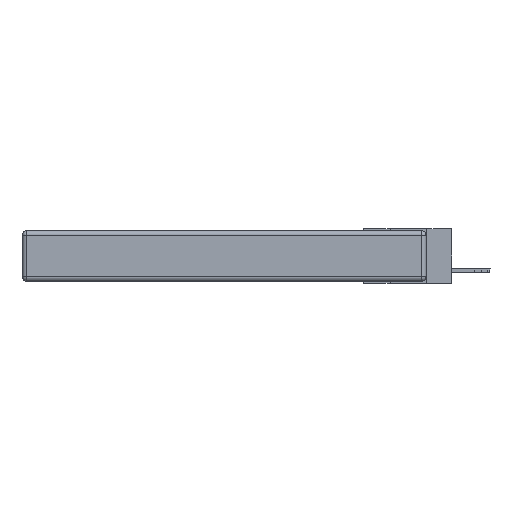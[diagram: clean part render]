
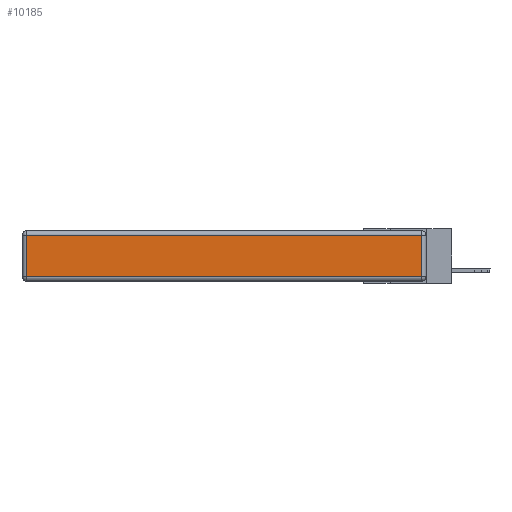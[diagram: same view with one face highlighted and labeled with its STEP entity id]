
A CAD part, left-side view. The second image highlights one B-rep face of the part: STEP entity #10185.
In plain terms, the highlighted planar face has unit normal (-1, 0, 0).
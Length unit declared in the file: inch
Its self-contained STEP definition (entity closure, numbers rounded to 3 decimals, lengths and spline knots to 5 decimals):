
#319 = LINE ( 'NONE', #3520, #14723 ) ;
#1107 = CARTESIAN_POINT ( 'NONE',  ( 0., 0., -0.343 ) ) ;
#1372 = ORIENTED_EDGE ( 'NONE', *, *, #13783, .T. ) ;
#1484 = VERTEX_POINT ( 'NONE', #5855 ) ;
#1899 = DIRECTION ( 'NONE',  ( 0., 0., 1. ) ) ;
#3520 = CARTESIAN_POINT ( 'NONE',  ( 0., 0., -0.313 ) ) ;
#4448 = FACE_OUTER_BOUND ( 'NONE', #14751, .T. ) ;
#4524 = VECTOR ( 'NONE', #13594, 39.37008 ) ;
#5392 = ORIENTED_EDGE ( 'NONE', *, *, #12137, .T. ) ;
#5855 = CARTESIAN_POINT ( 'NONE',  ( 0., 2.72, -0.313 ) ) ;
#6175 = EDGE_CURVE ( 'NONE', #1484, #7111, #319, .T. ) ;
#6207 = VECTOR ( 'NONE', #1899, 39.37008 ) ;
#6519 = CARTESIAN_POINT ( 'NONE',  ( 0., 2.72, -0.343 ) ) ;
#7111 = VERTEX_POINT ( 'NONE', #8872 ) ;
#7635 = ORIENTED_EDGE ( 'NONE', *, *, #6175, .T. ) ;
#7866 = DIRECTION ( 'NONE',  ( 0., -1., 0. ) ) ;
#8240 = PLANE ( 'NONE',  #17316 ) ;
#8872 = CARTESIAN_POINT ( 'NONE',  ( 0., 0.03, -0.313 ) ) ;
#9750 = DIRECTION ( 'NONE',  ( 0., 0., 1. ) ) ;
#9871 = DIRECTION ( 'NONE',  ( -1., 0., 0. ) ) ;
#10183 = CARTESIAN_POINT ( 'NONE',  ( 0., 0.03, -0.343 ) ) ;
#10185 = ADVANCED_FACE ( 'NONE', ( #4448 ), #8240, .T. ) ;
#10263 = CARTESIAN_POINT ( 'NONE',  ( 0., 2.75, -0.03 ) ) ;
#10469 = CARTESIAN_POINT ( 'NONE',  ( 0., 2.72, -0.03 ) ) ;
#10532 = ORIENTED_EDGE ( 'NONE', *, *, #17698, .T. ) ;
#10717 = LINE ( 'NONE', #10263, #11590 ) ;
#11590 = VECTOR ( 'NONE', #14641, 39.37008 ) ;
#12137 = EDGE_CURVE ( 'NONE', #14840, #13483, #10717, .T. ) ;
#12751 = LINE ( 'NONE', #10183, #6207 ) ;
#13483 = VERTEX_POINT ( 'NONE', #10469 ) ;
#13594 = DIRECTION ( 'NONE',  ( 0., 0., -1. ) ) ;
#13783 = EDGE_CURVE ( 'NONE', #13483, #1484, #15002, .T. ) ;
#14559 = CARTESIAN_POINT ( 'NONE',  ( 0., 0.03, -0.03 ) ) ;
#14641 = DIRECTION ( 'NONE',  ( 0., 1., 0. ) ) ;
#14723 = VECTOR ( 'NONE', #7866, 39.37008 ) ;
#14751 = EDGE_LOOP ( 'NONE', ( #7635, #10532, #5392, #1372 ) ) ;
#14840 = VERTEX_POINT ( 'NONE', #14559 ) ;
#15002 = LINE ( 'NONE', #6519, #4524 ) ;
#17316 = AXIS2_PLACEMENT_3D ( 'NONE', #1107, #9871, #9750 ) ;
#17698 = EDGE_CURVE ( 'NONE', #7111, #14840, #12751, .T. ) ;
